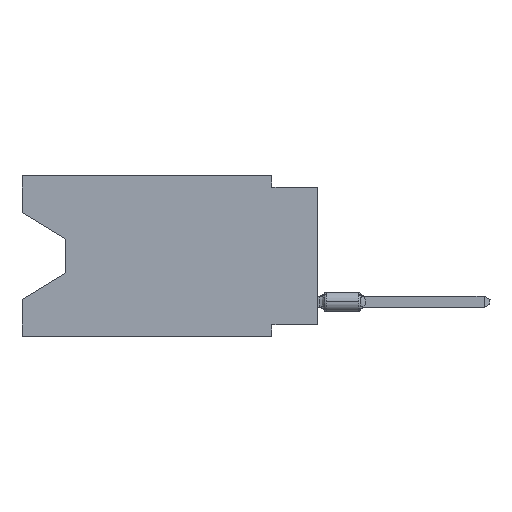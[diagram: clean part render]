
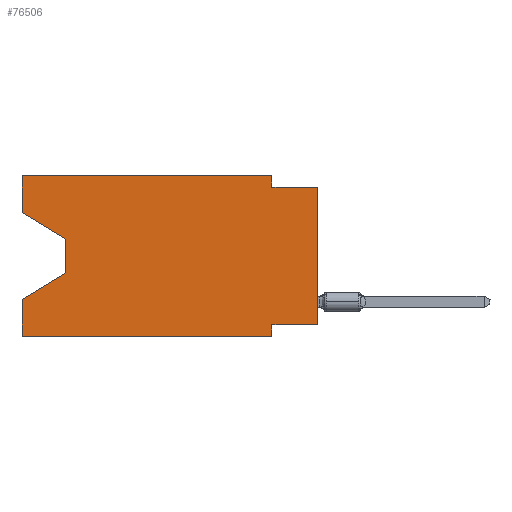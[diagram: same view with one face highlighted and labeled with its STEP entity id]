
A CAD part, left-side view. The second image highlights one B-rep face of the part: STEP entity #76506.
In plain terms, the highlighted planar face has unit normal (-1, 0, 0).
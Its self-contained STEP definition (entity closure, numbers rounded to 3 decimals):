
#676 = CARTESIAN_POINT ( 'NONE',  ( 0., 16.383, -2.038 ) ) ;
#1699 = ORIENTED_EDGE ( 'NONE', *, *, #81918, .T. ) ;
#2437 = VECTOR ( 'NONE', #60077, 1000. ) ;
#3400 = CARTESIAN_POINT ( 'NONE',  ( 0., 13.97, -5.385 ) ) ;
#3448 = CARTESIAN_POINT ( 'NONE',  ( 0., 0., -8.255 ) ) ;
#3469 = CARTESIAN_POINT ( 'NONE',  ( 0., 16.383, -8.89 ) ) ;
#3783 = EDGE_CURVE ( 'NONE', #78245, #38553, #38357, .T. ) ;
#4096 = EDGE_CURVE ( 'NONE', #13143, #41540, #10603, .T. ) ;
#6157 = ORIENTED_EDGE ( 'NONE', *, *, #3783, .F. ) ;
#6448 = CARTESIAN_POINT ( 'NONE',  ( 0., 16.383, -6.852 ) ) ;
#6611 = DIRECTION ( 'NONE',  ( 1., 0., 0. ) ) ;
#8142 = CARTESIAN_POINT ( 'NONE',  ( 0., 13.97, -3.505 ) ) ;
#9368 = CARTESIAN_POINT ( 'NONE',  ( 0., 13.97, -5.385 ) ) ;
#9857 = ORIENTED_EDGE ( 'NONE', *, *, #48182, .T. ) ;
#9940 = CARTESIAN_POINT ( 'NONE',  ( 0., 13.97, -3.505 ) ) ;
#10176 = DIRECTION ( 'NONE',  ( 0., -1., 0. ) ) ;
#10603 = LINE ( 'NONE', #3469, #73321 ) ;
#10878 = LINE ( 'NONE', #67962, #42240 ) ;
#11387 = ORIENTED_EDGE ( 'NONE', *, *, #71228, .T. ) ;
#12095 = VECTOR ( 'NONE', #19688, 1000. ) ;
#13143 = VERTEX_POINT ( 'NONE', #62592 ) ;
#13807 = VERTEX_POINT ( 'NONE', #25433 ) ;
#14552 = EDGE_CURVE ( 'NONE', #46216, #74929, #60978, .T. ) ;
#14831 = LINE ( 'NONE', #9368, #72180 ) ;
#17559 = VERTEX_POINT ( 'NONE', #57979 ) ;
#18383 = DIRECTION ( 'NONE',  ( 0., 0., 1. ) ) ;
#18963 = VERTEX_POINT ( 'NONE', #6448 ) ;
#19468 = LINE ( 'NONE', #8142, #80343 ) ;
#19688 = DIRECTION ( 'NONE',  ( 0., -1., 0. ) ) ;
#21545 = FACE_OUTER_BOUND ( 'NONE', #52614, .T. ) ;
#23732 = LINE ( 'NONE', #74969, #71339 ) ;
#24519 = DIRECTION ( 'NONE',  ( 0., -1., 0. ) ) ;
#24752 = ORIENTED_EDGE ( 'NONE', *, *, #48357, .F. ) ;
#25433 = CARTESIAN_POINT ( 'NONE',  ( 0., 0., -0.635 ) ) ;
#26342 = CARTESIAN_POINT ( 'NONE',  ( 0., 2.54, 0. ) ) ;
#26738 = LINE ( 'NONE', #77142, #29098 ) ;
#29098 = VECTOR ( 'NONE', #18383, 1000. ) ;
#33026 = DIRECTION ( 'NONE',  ( 0., 0., 1. ) ) ;
#34129 = PLANE ( 'NONE',  #69741 ) ;
#34967 = CARTESIAN_POINT ( 'NONE',  ( 0., 16.383, 0. ) ) ;
#36912 = VECTOR ( 'NONE', #44010, 1000. ) ;
#37946 = CARTESIAN_POINT ( 'NONE',  ( 0., 16.383, 0. ) ) ;
#38357 = LINE ( 'NONE', #37946, #54314 ) ;
#38366 = DIRECTION ( 'NONE',  ( 0., 0., -1. ) ) ;
#38553 = VERTEX_POINT ( 'NONE', #44533 ) ;
#40438 = DIRECTION ( 'NONE',  ( 0., 0., -1. ) ) ;
#41540 = VERTEX_POINT ( 'NONE', #64978 ) ;
#42240 = VECTOR ( 'NONE', #69203, 1000. ) ;
#42900 = VERTEX_POINT ( 'NONE', #9940 ) ;
#44010 = DIRECTION ( 'NONE',  ( 0., 0., -1. ) ) ;
#44533 = CARTESIAN_POINT ( 'NONE',  ( 0., 2.54, 0. ) ) ;
#45231 = LINE ( 'NONE', #64574, #79138 ) ;
#45823 = ORIENTED_EDGE ( 'NONE', *, *, #82102, .T. ) ;
#46216 = VERTEX_POINT ( 'NONE', #73305 ) ;
#48182 = EDGE_CURVE ( 'NONE', #58947, #42900, #10878, .T. ) ;
#48357 = EDGE_CURVE ( 'NONE', #38553, #17559, #62934, .T. ) ;
#50950 = ORIENTED_EDGE ( 'NONE', *, *, #78048, .F. ) ;
#52614 = EDGE_LOOP ( 'NONE', ( #9857, #1699, #45823, #73634, #58841, #50950, #66308, #11387, #74462, #24752, #6157, #55595 ) ) ;
#54314 = VECTOR ( 'NONE', #24519, 1000. ) ;
#54617 = LINE ( 'NONE', #61325, #2437 ) ;
#55595 = ORIENTED_EDGE ( 'NONE', *, *, #55745, .F. ) ;
#55745 = EDGE_CURVE ( 'NONE', #58947, #78245, #45231, .T. ) ;
#57979 = CARTESIAN_POINT ( 'NONE',  ( 0., 2.54, -0.635 ) ) ;
#58841 = ORIENTED_EDGE ( 'NONE', *, *, #4096, .T. ) ;
#58947 = VERTEX_POINT ( 'NONE', #676 ) ;
#60077 = DIRECTION ( 'NONE',  ( 0., 0., 1. ) ) ;
#60595 = DIRECTION ( 'NONE',  ( 0., 0.855, -0.519 ) ) ;
#60978 = LINE ( 'NONE', #3448, #75926 ) ;
#61325 = CARTESIAN_POINT ( 'NONE',  ( 0., 16.383, 0. ) ) ;
#61487 = VERTEX_POINT ( 'NONE', #3400 ) ;
#62592 = CARTESIAN_POINT ( 'NONE',  ( 0., 16.383, -8.89 ) ) ;
#62934 = LINE ( 'NONE', #26342, #36912 ) ;
#64574 = CARTESIAN_POINT ( 'NONE',  ( 0., 16.383, 0. ) ) ;
#64978 = CARTESIAN_POINT ( 'NONE',  ( 0., 2.54, -8.89 ) ) ;
#66308 = ORIENTED_EDGE ( 'NONE', *, *, #14552, .F. ) ;
#67962 = CARTESIAN_POINT ( 'NONE',  ( 0., 16.383, -2.038 ) ) ;
#69203 = DIRECTION ( 'NONE',  ( 0., -0.855, -0.519 ) ) ;
#69479 = CARTESIAN_POINT ( 'NONE',  ( 0., 2.54, -8.255 ) ) ;
#69741 = AXIS2_PLACEMENT_3D ( 'NONE', #34967, #6611, #40438 ) ;
#71228 = EDGE_CURVE ( 'NONE', #46216, #13807, #26738, .T. ) ;
#71339 = VECTOR ( 'NONE', #81669, 1000. ) ;
#72147 = LINE ( 'NONE', #78039, #12095 ) ;
#72180 = VECTOR ( 'NONE', #60595, 1000. ) ;
#73305 = CARTESIAN_POINT ( 'NONE',  ( 0., 0., -8.255 ) ) ;
#73321 = VECTOR ( 'NONE', #10176, 1000. ) ;
#73634 = ORIENTED_EDGE ( 'NONE', *, *, #74274, .F. ) ;
#74274 = EDGE_CURVE ( 'NONE', #13143, #18963, #54617, .T. ) ;
#74462 = ORIENTED_EDGE ( 'NONE', *, *, #76100, .F. ) ;
#74929 = VERTEX_POINT ( 'NONE', #69479 ) ;
#74969 = CARTESIAN_POINT ( 'NONE',  ( 0., 2.54, -8.89 ) ) ;
#75926 = VECTOR ( 'NONE', #80264, 1000. ) ;
#76100 = EDGE_CURVE ( 'NONE', #17559, #13807, #72147, .T. ) ;
#76506 = ADVANCED_FACE ( 'NONE', ( #21545 ), #34129, .F. ) ;
#77142 = CARTESIAN_POINT ( 'NONE',  ( 0., 0., 0. ) ) ;
#78039 = CARTESIAN_POINT ( 'NONE',  ( 0., 0., -0.635 ) ) ;
#78048 = EDGE_CURVE ( 'NONE', #74929, #41540, #23732, .T. ) ;
#78245 = VERTEX_POINT ( 'NONE', #79505 ) ;
#79138 = VECTOR ( 'NONE', #33026, 1000. ) ;
#79505 = CARTESIAN_POINT ( 'NONE',  ( 0., 16.383, 0. ) ) ;
#80264 = DIRECTION ( 'NONE',  ( 0., 1., 0. ) ) ;
#80343 = VECTOR ( 'NONE', #38366, 1000. ) ;
#81669 = DIRECTION ( 'NONE',  ( 0., 0., -1. ) ) ;
#81918 = EDGE_CURVE ( 'NONE', #42900, #61487, #19468, .T. ) ;
#82102 = EDGE_CURVE ( 'NONE', #61487, #18963, #14831, .T. ) ;
